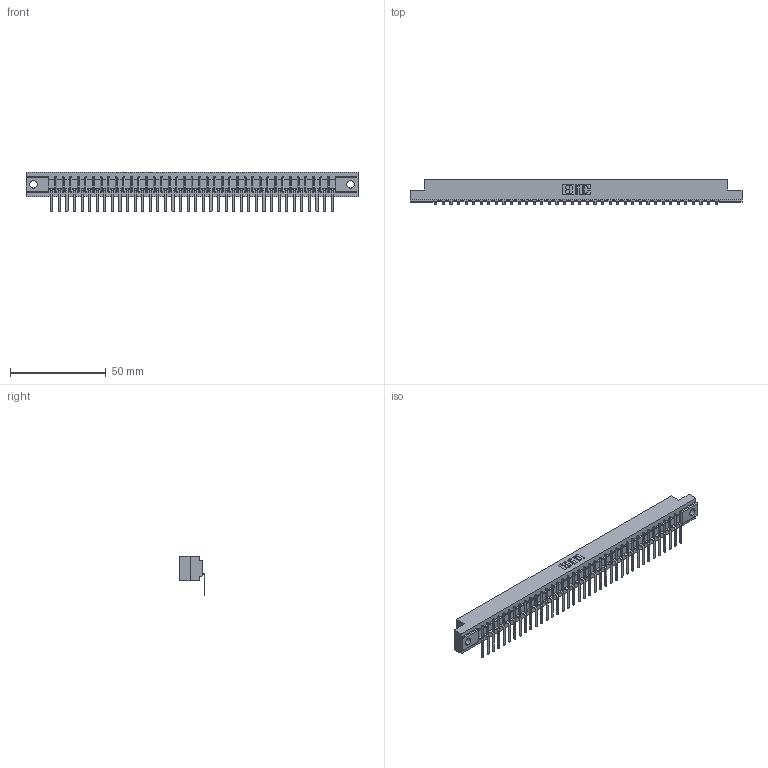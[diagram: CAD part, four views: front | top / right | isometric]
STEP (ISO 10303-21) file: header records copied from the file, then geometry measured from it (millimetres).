
FILE_DESCRIPTION (( 'STEP AP203' ), '1' );
FILE_NAME ('307-038-457-104.STEP', '2020-09-29T06:45:32', ( '' ), ( '' ), 'SwSTEP 2.0', 'SolidWorks 2020', '' );
FILE_SCHEMA (( 'CONFIG_CONTROL_DESIGN' ));
Length unit declared in the file: inch
Products named in the file (3): 307-038-457-104; 307-290-002_557; 307 Part_.156 Dia Mounting Holes
Assembly tree (39 placements, depth 2):
  307-038-457-104
    307 Part_.156 Dia Mounting Holes
    307-290-002_557  x38
Bounding box: 173.58 x 13.32 x 20.66 mm (x, y, z)
Volume: 18542.4 mm3; surface area: 23729.2 mm2
Topology: 39 solids, 39 shells, 3135 faces, 9631 edges, 6314 vertices
Faces by surface type: plane 1870, cylinder 1187, sphere 78
Entity records: 34342 total; most frequent: CARTESIAN_POINT 5798, ORIENTED_EDGE 5786, DIRECTION 5627, EDGE_CURVE 2893, LINE 2221, VECTOR 2221, VERTEX_POINT 1874, AXIS2_PLACEMENT_3D 1703
